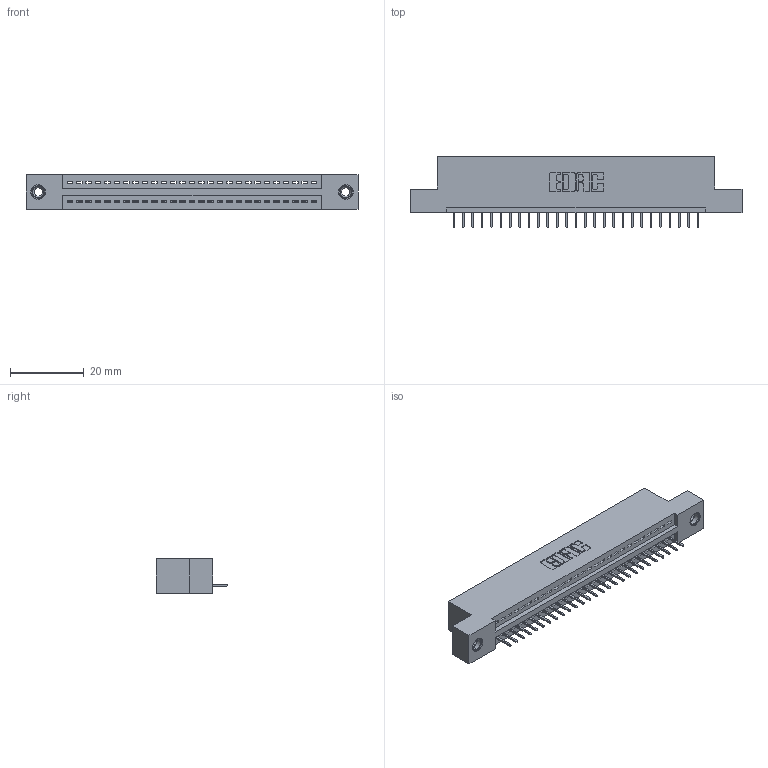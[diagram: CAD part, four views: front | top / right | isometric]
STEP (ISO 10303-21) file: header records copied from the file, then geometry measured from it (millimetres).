
FILE_DESCRIPTION (( 'STEP AP203' ), '1' );
FILE_NAME ('345-027-524-108.STEP', '2018-08-22T05:29:29', ( '' ), ( '' ), 'SwSTEP 2.0', 'SolidWorks 2016', '' );
FILE_SCHEMA (( 'CONFIG_CONTROL_DESIGN' ));
Length unit declared in the file: inch
Products named in the file (4): 345 Part_Flush Mounting Lugs - 0.156 Dia-TI; 345-292-001_345-293-124; 345-250-001_345-250-003-102; 345-027-524-108
Assembly tree (30 placements, depth 2):
  345-027-524-108
    345 Part_Flush Mounting Lugs - 0.156 Dia-TI
    345-292-001_345-293-124  x27
    345-250-001_345-250-003-102  x2
Bounding box: 89.79 x 19.35 x 9.4 mm (x, y, z)
Volume: 8292.2 mm3; surface area: 10493.8 mm2
Topology: 30 solids, 30 shells, 1860 faces, 5337 edges, 3442 vertices
Faces by surface type: plane 1354, cylinder 490, cone 12, torus 4
Entity records: 23600 total; most frequent: CARTESIAN_POINT 4068, ORIENTED_EDGE 4022, DIRECTION 3603, EDGE_CURVE 2011, VECTOR 1755, LINE 1755, VERTEX_POINT 1332, AXIS2_PLACEMENT_3D 924
